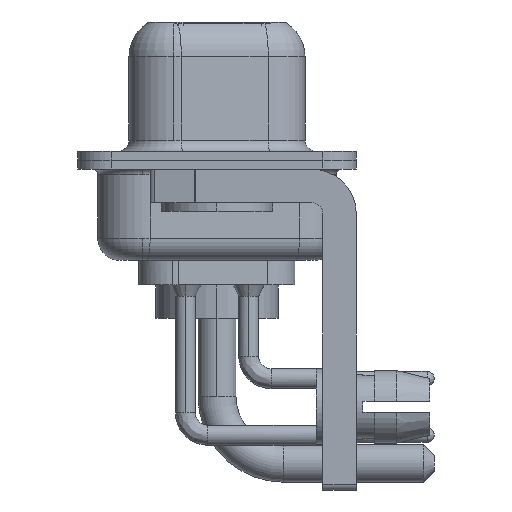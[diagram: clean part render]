
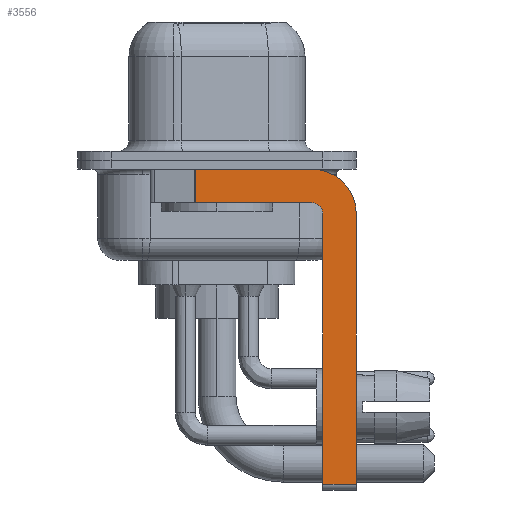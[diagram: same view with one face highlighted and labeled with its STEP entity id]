
A CAD part, left-side view. The second image highlights one B-rep face of the part: STEP entity #3556.
In plain terms, the highlighted planar face has unit normal (-1, 0, 0).
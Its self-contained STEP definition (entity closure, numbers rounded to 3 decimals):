
#337 = VECTOR ( 'NONE', #12227, 1000. ) ;
#850 = DIRECTION ( 'NONE',  ( 0., 1., 0. ) ) ;
#1349 = ORIENTED_EDGE ( 'NONE', *, *, #10882, .T. ) ;
#1489 = ORIENTED_EDGE ( 'NONE', *, *, #19008, .F. ) ;
#1503 = VERTEX_POINT ( 'NONE', #11051 ) ;
#1655 = CIRCLE ( 'NONE', #9134, 2. ) ;
#1660 = CARTESIAN_POINT ( 'NONE',  ( -2.9, 3., -0.4 ) ) ;
#1714 = DIRECTION ( 'NONE',  ( 0., 0., 1. ) ) ;
#2247 = ORIENTED_EDGE ( 'NONE', *, *, #8153, .F. ) ;
#2895 = VERTEX_POINT ( 'NONE', #19975 ) ;
#3108 = CARTESIAN_POINT ( 'NONE',  ( -2.9, -4.75, -14.55 ) ) ;
#3465 = VECTOR ( 'NONE', #5437, 1000. ) ;
#3556 = ADVANCED_FACE ( 'NONE', ( #9173 ), #15639, .F. ) ;
#3569 = AXIS2_PLACEMENT_3D ( 'NONE', #13541, #17558, #17346 ) ;
#3691 = AXIS2_PLACEMENT_3D ( 'NONE', #16385, #8028, #1714 ) ;
#3933 = EDGE_CURVE ( 'NONE', #1503, #17496, #17323, .T. ) ;
#4034 = ORIENTED_EDGE ( 'NONE', *, *, #20122, .F. ) ;
#4451 = EDGE_CURVE ( 'NONE', #2895, #15094, #12833, .T. ) ;
#4532 = EDGE_CURVE ( 'NONE', #9525, #6147, #6271, .T. ) ;
#5437 = DIRECTION ( 'NONE',  ( 0., -1., 0. ) ) ;
#5765 = LINE ( 'NONE', #15086, #337 ) ;
#6147 = VERTEX_POINT ( 'NONE', #19090 ) ;
#6271 = LINE ( 'NONE', #1660, #13749 ) ;
#6769 = ORIENTED_EDGE ( 'NONE', *, *, #4532, .F. ) ;
#7045 = CARTESIAN_POINT ( 'NONE',  ( -2.9, -4.25, -14.55 ) ) ;
#7414 = CARTESIAN_POINT ( 'NONE',  ( -2.9, -4.75, -14.8 ) ) ;
#7633 = LINE ( 'NONE', #7414, #13232 ) ;
#8028 = DIRECTION ( 'NONE',  ( -1., 0., 0. ) ) ;
#8153 = EDGE_CURVE ( 'NONE', #11421, #1503, #13527, .T. ) ;
#8527 = ORIENTED_EDGE ( 'NONE', *, *, #12296, .T. ) ;
#8665 = VECTOR ( 'NONE', #850, 1000. ) ;
#8736 = LINE ( 'NONE', #7045, #3465 ) ;
#8847 = ORIENTED_EDGE ( 'NONE', *, *, #3933, .F. ) ;
#9134 = AXIS2_PLACEMENT_3D ( 'NONE', #12990, #19600, #19498 ) ;
#9173 = FACE_OUTER_BOUND ( 'NONE', #20257, .T. ) ;
#9525 = VERTEX_POINT ( 'NONE', #19209 ) ;
#9857 = DIRECTION ( 'NONE',  ( 0., -1., 0. ) ) ;
#10882 = EDGE_CURVE ( 'NONE', #9525, #17496, #5765, .T. ) ;
#11033 = DIRECTION ( 'NONE',  ( 0., 0., -1. ) ) ;
#11051 = CARTESIAN_POINT ( 'NONE',  ( -2.9, -4.25, -1.9 ) ) ;
#11208 = CARTESIAN_POINT ( 'NONE',  ( -2.9, 0.978, -1.9 ) ) ;
#11421 = VERTEX_POINT ( 'NONE', #15987 ) ;
#12227 = DIRECTION ( 'NONE',  ( 0., 0., -1. ) ) ;
#12296 = EDGE_CURVE ( 'NONE', #15868, #15094, #8736, .T. ) ;
#12833 = LINE ( 'NONE', #19336, #20576 ) ;
#12990 = CARTESIAN_POINT ( 'NONE',  ( -2.9, -4.25, -2.4 ) ) ;
#13232 = VECTOR ( 'NONE', #15779, 1000. ) ;
#13527 = CIRCLE ( 'NONE', #3691, 0.5 ) ;
#13541 = CARTESIAN_POINT ( 'NONE',  ( -2.9, -4.25, -2.4 ) ) ;
#13749 = VECTOR ( 'NONE', #9857, 1000. ) ;
#15086 = CARTESIAN_POINT ( 'NONE',  ( -2.9, 0.978, -1.9 ) ) ;
#15094 = VERTEX_POINT ( 'NONE', #19351 ) ;
#15639 = PLANE ( 'NONE',  #3569 ) ;
#15729 = CARTESIAN_POINT ( 'NONE',  ( -2.9, -4.25, -1.9 ) ) ;
#15779 = DIRECTION ( 'NONE',  ( 0., 0., 1. ) ) ;
#15868 = VERTEX_POINT ( 'NONE', #3108 ) ;
#15987 = CARTESIAN_POINT ( 'NONE',  ( -2.9, -4.75, -2.4 ) ) ;
#16385 = CARTESIAN_POINT ( 'NONE',  ( -2.9, -4.25, -2.4 ) ) ;
#17323 = LINE ( 'NONE', #15729, #8665 ) ;
#17346 = DIRECTION ( 'NONE',  ( 0., 0., -1. ) ) ;
#17496 = VERTEX_POINT ( 'NONE', #11208 ) ;
#17558 = DIRECTION ( 'NONE',  ( 1., 0., 0. ) ) ;
#19008 = EDGE_CURVE ( 'NONE', #6147, #2895, #1655, .T. ) ;
#19090 = CARTESIAN_POINT ( 'NONE',  ( -2.9, -4.25, -0.4 ) ) ;
#19209 = CARTESIAN_POINT ( 'NONE',  ( -2.9, 0.978, -0.4 ) ) ;
#19336 = CARTESIAN_POINT ( 'NONE',  ( -2.9, -6.25, -2.4 ) ) ;
#19351 = CARTESIAN_POINT ( 'NONE',  ( -2.9, -6.25, -14.55 ) ) ;
#19498 = DIRECTION ( 'NONE',  ( 0., 0., -1. ) ) ;
#19600 = DIRECTION ( 'NONE',  ( 1., 0., 0. ) ) ;
#19975 = CARTESIAN_POINT ( 'NONE',  ( -2.9, -6.25, -2.4 ) ) ;
#19992 = ORIENTED_EDGE ( 'NONE', *, *, #4451, .F. ) ;
#20122 = EDGE_CURVE ( 'NONE', #15868, #11421, #7633, .T. ) ;
#20257 = EDGE_LOOP ( 'NONE', ( #6769, #1349, #8847, #2247, #4034, #8527, #19992, #1489 ) ) ;
#20576 = VECTOR ( 'NONE', #11033, 1000. ) ;
